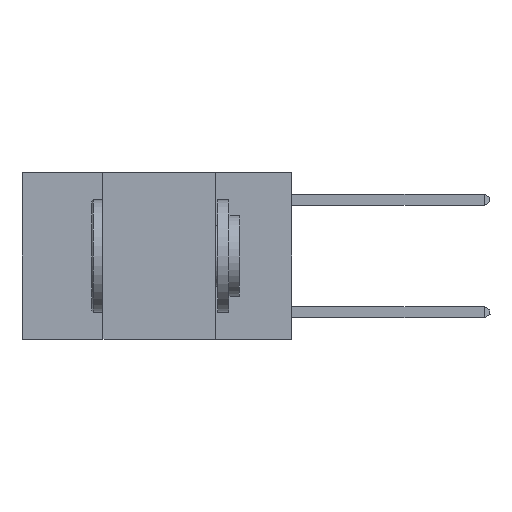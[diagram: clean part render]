
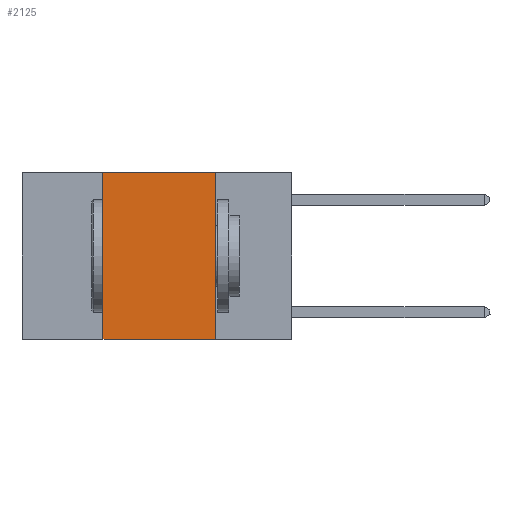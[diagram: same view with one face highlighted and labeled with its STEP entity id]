
A CAD part, left-side view. The second image highlights one B-rep face of the part: STEP entity #2125.
In plain terms, the highlighted planar face has unit normal (-1, 0, 0).
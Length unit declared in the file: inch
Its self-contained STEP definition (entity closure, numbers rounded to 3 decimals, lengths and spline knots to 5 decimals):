
#559 = LINE ( 'NONE', #9033, #3122 ) ;
#601 = EDGE_CURVE ( 'NONE', #5292, #8733, #3996, .T. ) ;
#672 = VERTEX_POINT ( 'NONE', #12649 ) ;
#1040 = VECTOR ( 'NONE', #2940, 39.37008 ) ;
#1555 = CARTESIAN_POINT ( 'NONE',  ( 0., 0.17, 0. ) ) ;
#2063 = EDGE_CURVE ( 'NONE', #8002, #5292, #5089, .T. ) ;
#2125 = ADVANCED_FACE ( 'NONE', ( #11515 ), #4577, .F. ) ;
#2449 = LINE ( 'NONE', #5992, #7674 ) ;
#2597 = CARTESIAN_POINT ( 'NONE',  ( 0., 0.6, 0. ) ) ;
#2777 = AXIS2_PLACEMENT_3D ( 'NONE', #10634, #5611, #12560 ) ;
#2940 = DIRECTION ( 'NONE',  ( 0., -1., 0. ) ) ;
#3122 = VECTOR ( 'NONE', #8060, 39.37008 ) ;
#3319 = CARTESIAN_POINT ( 'NONE',  ( 0., 0.42, 0. ) ) ;
#3465 = ORIENTED_EDGE ( 'NONE', *, *, #4322, .F. ) ;
#3536 = ORIENTED_EDGE ( 'NONE', *, *, #5681, .T. ) ;
#3996 = LINE ( 'NONE', #2597, #1040 ) ;
#4247 = ORIENTED_EDGE ( 'NONE', *, *, #601, .F. ) ;
#4322 = EDGE_CURVE ( 'NONE', #8733, #672, #2449, .T. ) ;
#4459 = ORIENTED_EDGE ( 'NONE', *, *, #2063, .F. ) ;
#4577 = PLANE ( 'NONE',  #2777 ) ;
#5089 = LINE ( 'NONE', #3319, #12694 ) ;
#5292 = VERTEX_POINT ( 'NONE', #5495 ) ;
#5495 = CARTESIAN_POINT ( 'NONE',  ( 0., 0.42, 0. ) ) ;
#5611 = DIRECTION ( 'NONE',  ( 1., 0., 0. ) ) ;
#5681 = EDGE_CURVE ( 'NONE', #8002, #672, #559, .T. ) ;
#5992 = CARTESIAN_POINT ( 'NONE',  ( 0., 0.17, 0. ) ) ;
#7413 = DIRECTION ( 'NONE',  ( 0., 0., 1. ) ) ;
#7674 = VECTOR ( 'NONE', #11995, 39.37008 ) ;
#8002 = VERTEX_POINT ( 'NONE', #10737 ) ;
#8060 = DIRECTION ( 'NONE',  ( 0., -1., 0. ) ) ;
#8733 = VERTEX_POINT ( 'NONE', #1555 ) ;
#9033 = CARTESIAN_POINT ( 'NONE',  ( 0., 0.6, -0.37 ) ) ;
#9112 = EDGE_LOOP ( 'NONE', ( #3465, #4247, #4459, #3536 ) ) ;
#10634 = CARTESIAN_POINT ( 'NONE',  ( 0., 0.6, 0. ) ) ;
#10737 = CARTESIAN_POINT ( 'NONE',  ( 0., 0.42, -0.37 ) ) ;
#11515 = FACE_OUTER_BOUND ( 'NONE', #9112, .T. ) ;
#11995 = DIRECTION ( 'NONE',  ( 0., 0., -1. ) ) ;
#12560 = DIRECTION ( 'NONE',  ( 0., 0., -1. ) ) ;
#12649 = CARTESIAN_POINT ( 'NONE',  ( 0., 0.17, -0.37 ) ) ;
#12694 = VECTOR ( 'NONE', #7413, 39.37008 ) ;
